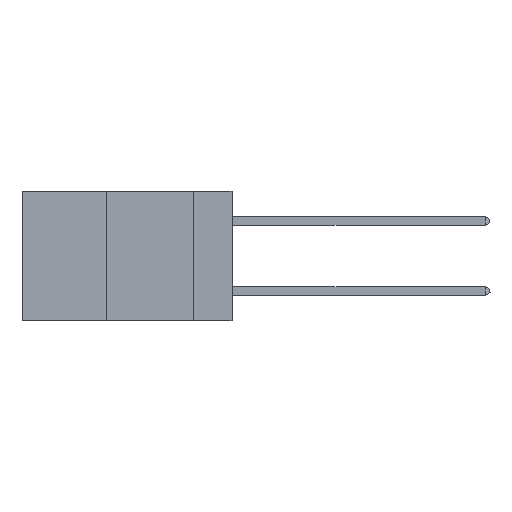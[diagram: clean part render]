
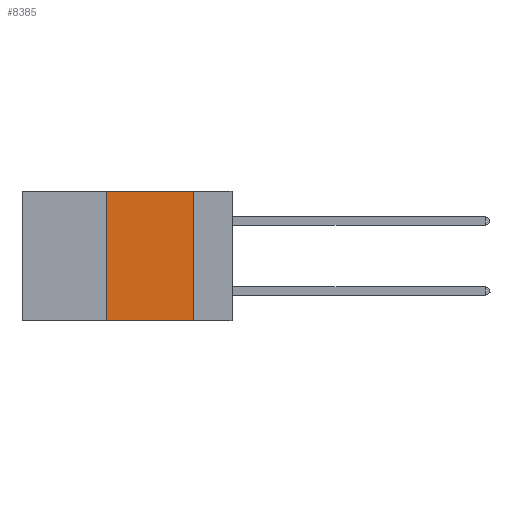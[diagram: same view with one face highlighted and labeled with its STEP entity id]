
A CAD part, left-side view. The second image highlights one B-rep face of the part: STEP entity #8385.
In plain terms, the highlighted planar face has unit normal (-1, 0, 0).
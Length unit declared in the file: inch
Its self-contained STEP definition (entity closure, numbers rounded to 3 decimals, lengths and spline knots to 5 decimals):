
#46 = CARTESIAN_POINT ( 'NONE',  ( 0., 0.11, 0. ) ) ;
#522 = EDGE_CURVE ( 'NONE', #2602, #10433, #4343, .T. ) ;
#1002 = EDGE_CURVE ( 'NONE', #10433, #4831, #10383, .T. ) ;
#1094 = CARTESIAN_POINT ( 'NONE',  ( 0., 0.11, -0.37 ) ) ;
#1435 = CARTESIAN_POINT ( 'NONE',  ( 0., 0.36, -0.37 ) ) ;
#1941 = PLANE ( 'NONE',  #4854 ) ;
#2141 = EDGE_CURVE ( 'NONE', #6412, #2602, #7311, .T. ) ;
#2602 = VERTEX_POINT ( 'NONE', #7041 ) ;
#2666 = CARTESIAN_POINT ( 'NONE',  ( 0., 0.36, 0. ) ) ;
#3337 = CARTESIAN_POINT ( 'NONE',  ( 0., 0.11, 0. ) ) ;
#3764 = CARTESIAN_POINT ( 'NONE',  ( 0., 0.6, -0.37 ) ) ;
#3778 = DIRECTION ( 'NONE',  ( 1., 0., 0. ) ) ;
#3804 = DIRECTION ( 'NONE',  ( 0., -1., 0. ) ) ;
#4343 = LINE ( 'NONE', #5298, #8872 ) ;
#4554 = DIRECTION ( 'NONE',  ( 0., 0., -1. ) ) ;
#4831 = VERTEX_POINT ( 'NONE', #1094 ) ;
#4854 = AXIS2_PLACEMENT_3D ( 'NONE', #9812, #3778, #4554 ) ;
#4993 = ORIENTED_EDGE ( 'NONE', *, *, #522, .F. ) ;
#5023 = VECTOR ( 'NONE', #7150, 39.37008 ) ;
#5298 = CARTESIAN_POINT ( 'NONE',  ( 0., 0.6, 0. ) ) ;
#5555 = VECTOR ( 'NONE', #3804, 39.37008 ) ;
#6412 = VERTEX_POINT ( 'NONE', #1435 ) ;
#6671 = FACE_OUTER_BOUND ( 'NONE', #10965, .T. ) ;
#7041 = CARTESIAN_POINT ( 'NONE',  ( 0., 0.36, 0. ) ) ;
#7150 = DIRECTION ( 'NONE',  ( 0., 0., -1. ) ) ;
#7223 = DIRECTION ( 'NONE',  ( 0., 0., 1. ) ) ;
#7311 = LINE ( 'NONE', #2666, #9805 ) ;
#7944 = ORIENTED_EDGE ( 'NONE', *, *, #11250, .T. ) ;
#8385 = ADVANCED_FACE ( 'NONE', ( #6671 ), #1941, .F. ) ;
#8750 = ORIENTED_EDGE ( 'NONE', *, *, #1002, .F. ) ;
#8872 = VECTOR ( 'NONE', #11445, 39.37008 ) ;
#9805 = VECTOR ( 'NONE', #7223, 39.37008 ) ;
#9812 = CARTESIAN_POINT ( 'NONE',  ( 0., 0.6, 0. ) ) ;
#10383 = LINE ( 'NONE', #46, #5023 ) ;
#10433 = VERTEX_POINT ( 'NONE', #3337 ) ;
#10899 = ORIENTED_EDGE ( 'NONE', *, *, #2141, .F. ) ;
#10965 = EDGE_LOOP ( 'NONE', ( #8750, #4993, #10899, #7944 ) ) ;
#11046 = LINE ( 'NONE', #3764, #5555 ) ;
#11250 = EDGE_CURVE ( 'NONE', #6412, #4831, #11046, .T. ) ;
#11445 = DIRECTION ( 'NONE',  ( 0., -1., 0. ) ) ;
